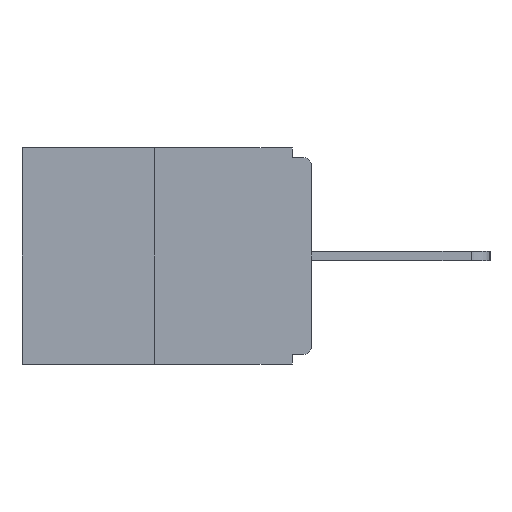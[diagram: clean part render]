
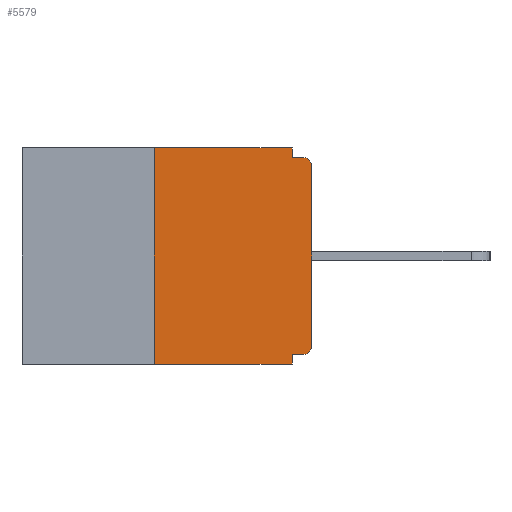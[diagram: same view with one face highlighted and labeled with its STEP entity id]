
A CAD part, left-side view. The second image highlights one B-rep face of the part: STEP entity #5579.
In plain terms, the highlighted planar face has unit normal (-1, 0, 0).
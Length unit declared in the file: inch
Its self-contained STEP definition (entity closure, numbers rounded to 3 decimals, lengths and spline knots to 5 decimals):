
#38 = CARTESIAN_POINT ( 'NONE',  ( 0., 0.46, -0.343 ) ) ;
#144 = VECTOR ( 'NONE', #8667, 39.37008 ) ;
#344 = CARTESIAN_POINT ( 'NONE',  ( 0., 0.031, -0.343 ) ) ;
#418 = VERTEX_POINT ( 'NONE', #8107 ) ;
#482 = DIRECTION ( 'NONE',  ( 0., 0., -1. ) ) ;
#510 = VERTEX_POINT ( 'NONE', #13588 ) ;
#606 = VERTEX_POINT ( 'NONE', #7046 ) ;
#672 = LINE ( 'NONE', #1011, #7446 ) ;
#1011 = CARTESIAN_POINT ( 'NONE',  ( 0., 0.25, 0. ) ) ;
#1106 = DIRECTION ( 'NONE',  ( 0., 0., -1. ) ) ;
#1250 = PLANE ( 'NONE',  #7319 ) ;
#1345 = CARTESIAN_POINT ( 'NONE',  ( 0., 0., -0.015 ) ) ;
#1381 = CARTESIAN_POINT ( 'NONE',  ( 0., 0.46, 0. ) ) ;
#1570 = EDGE_CURVE ( 'NONE', #606, #15795, #4738, .T. ) ;
#2025 = LINE ( 'NONE', #38, #11490 ) ;
#2544 = CIRCLE ( 'NONE', #13213, 0.015 ) ;
#2579 = EDGE_CURVE ( 'NONE', #11965, #510, #3741, .T. ) ;
#2638 = CARTESIAN_POINT ( 'NONE',  ( 0., 0.015, -0.313 ) ) ;
#2947 = DIRECTION ( 'NONE',  ( 1., 0., 0. ) ) ;
#3218 = DIRECTION ( 'NONE',  ( 0., -1., 0. ) ) ;
#3249 = CARTESIAN_POINT ( 'NONE',  ( 0., 0.46, 0. ) ) ;
#3520 = VERTEX_POINT ( 'NONE', #14445 ) ;
#3693 = ORIENTED_EDGE ( 'NONE', *, *, #9591, .F. ) ;
#3741 = LINE ( 'NONE', #1345, #9918 ) ;
#3870 = ORIENTED_EDGE ( 'NONE', *, *, #15872, .T. ) ;
#3879 = AXIS2_PLACEMENT_3D ( 'NONE', #7922, #7895, #7833 ) ;
#3924 = DIRECTION ( 'NONE',  ( 0., 0., -1. ) ) ;
#4012 = ORIENTED_EDGE ( 'NONE', *, *, #13361, .F. ) ;
#4052 = ORIENTED_EDGE ( 'NONE', *, *, #1570, .F. ) ;
#4717 = VERTEX_POINT ( 'NONE', #9017 ) ;
#4738 = LINE ( 'NONE', #3249, #14518 ) ;
#4795 = EDGE_CURVE ( 'NONE', #15795, #11965, #6944, .T. ) ;
#5124 = CARTESIAN_POINT ( 'NONE',  ( 0., 0., -0.03 ) ) ;
#5367 = ORIENTED_EDGE ( 'NONE', *, *, #4795, .F. ) ;
#5392 = VERTEX_POINT ( 'NONE', #13529 ) ;
#5476 = CIRCLE ( 'NONE', #3879, 0.015 ) ;
#5573 = ORIENTED_EDGE ( 'NONE', *, *, #2579, .F. ) ;
#5579 = ADVANCED_FACE ( 'NONE', ( #14955 ), #1250, .F. ) ;
#5622 = ORIENTED_EDGE ( 'NONE', *, *, #9032, .T. ) ;
#5830 = ORIENTED_EDGE ( 'NONE', *, *, #12789, .T. ) ;
#5848 = ORIENTED_EDGE ( 'NONE', *, *, #13509, .T. ) ;
#6119 = VECTOR ( 'NONE', #15907, 39.37008 ) ;
#6448 = EDGE_LOOP ( 'NONE', ( #4052, #4012, #3870, #3693, #6472, #5848, #5830, #5622, #5573, #5367 ) ) ;
#6472 = ORIENTED_EDGE ( 'NONE', *, *, #7874, .F. ) ;
#6944 = LINE ( 'NONE', #8679, #144 ) ;
#7046 = CARTESIAN_POINT ( 'NONE',  ( 0., 0.25, 0. ) ) ;
#7179 = CARTESIAN_POINT ( 'NONE',  ( 0., 0.031, -0.015 ) ) ;
#7319 = AXIS2_PLACEMENT_3D ( 'NONE', #1381, #2947, #1106 ) ;
#7446 = VECTOR ( 'NONE', #12183, 39.37008 ) ;
#7477 = CARTESIAN_POINT ( 'NONE',  ( 0., 0., 0. ) ) ;
#7833 = DIRECTION ( 'NONE',  ( 0., 0., -1. ) ) ;
#7874 = EDGE_CURVE ( 'NONE', #5392, #12822, #10108, .T. ) ;
#7895 = DIRECTION ( 'NONE',  ( -1., 0., 0. ) ) ;
#7922 = CARTESIAN_POINT ( 'NONE',  ( 0., 0.015, -0.03 ) ) ;
#8107 = CARTESIAN_POINT ( 'NONE',  ( 0., 0.25, -0.343 ) ) ;
#8667 = DIRECTION ( 'NONE',  ( 0., 0., -1. ) ) ;
#8679 = CARTESIAN_POINT ( 'NONE',  ( 0., 0.031, 0. ) ) ;
#8963 = DIRECTION ( 'NONE',  ( 0., -1., 0. ) ) ;
#9017 = CARTESIAN_POINT ( 'NONE',  ( 0., 0.031, -0.343 ) ) ;
#9032 = EDGE_CURVE ( 'NONE', #13487, #510, #5476, .T. ) ;
#9337 = VECTOR ( 'NONE', #482, 39.37008 ) ;
#9423 = LINE ( 'NONE', #7477, #6119 ) ;
#9591 = EDGE_CURVE ( 'NONE', #12822, #4717, #15714, .T. ) ;
#9918 = VECTOR ( 'NONE', #13891, 39.37008 ) ;
#10108 = LINE ( 'NONE', #11550, #13802 ) ;
#11171 = CARTESIAN_POINT ( 'NONE',  ( 0., 0.031, 0. ) ) ;
#11237 = DIRECTION ( 'NONE',  ( -1., 0., 0. ) ) ;
#11490 = VECTOR ( 'NONE', #8963, 39.37008 ) ;
#11513 = DIRECTION ( 'NONE',  ( 0., 1., 0. ) ) ;
#11550 = CARTESIAN_POINT ( 'NONE',  ( 0., 0., -0.328 ) ) ;
#11965 = VERTEX_POINT ( 'NONE', #7179 ) ;
#12183 = DIRECTION ( 'NONE',  ( 0., 0., 1. ) ) ;
#12789 = EDGE_CURVE ( 'NONE', #3520, #13487, #9423, .T. ) ;
#12822 = VERTEX_POINT ( 'NONE', #15955 ) ;
#13213 = AXIS2_PLACEMENT_3D ( 'NONE', #2638, #11237, #3924 ) ;
#13361 = EDGE_CURVE ( 'NONE', #418, #606, #672, .T. ) ;
#13487 = VERTEX_POINT ( 'NONE', #5124 ) ;
#13509 = EDGE_CURVE ( 'NONE', #5392, #3520, #2544, .T. ) ;
#13529 = CARTESIAN_POINT ( 'NONE',  ( 0., 0.015, -0.328 ) ) ;
#13588 = CARTESIAN_POINT ( 'NONE',  ( 0., 0.015, -0.015 ) ) ;
#13802 = VECTOR ( 'NONE', #11513, 39.37008 ) ;
#13891 = DIRECTION ( 'NONE',  ( 0., -1., 0. ) ) ;
#14445 = CARTESIAN_POINT ( 'NONE',  ( 0., 0., -0.313 ) ) ;
#14518 = VECTOR ( 'NONE', #3218, 39.37008 ) ;
#14955 = FACE_OUTER_BOUND ( 'NONE', #6448, .T. ) ;
#15714 = LINE ( 'NONE', #344, #9337 ) ;
#15795 = VERTEX_POINT ( 'NONE', #11171 ) ;
#15872 = EDGE_CURVE ( 'NONE', #418, #4717, #2025, .T. ) ;
#15907 = DIRECTION ( 'NONE',  ( 0., 0., 1. ) ) ;
#15955 = CARTESIAN_POINT ( 'NONE',  ( 0., 0.031, -0.328 ) ) ;
